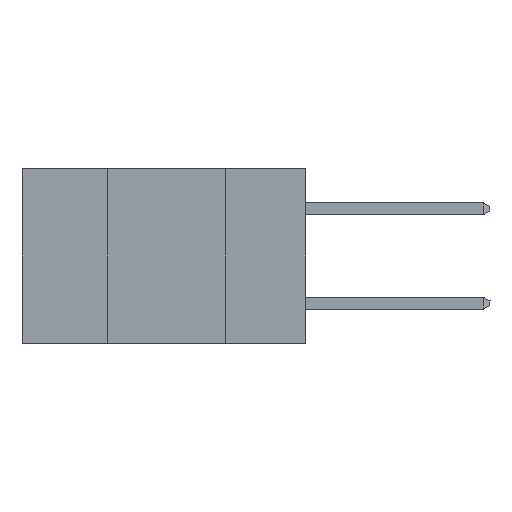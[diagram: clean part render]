
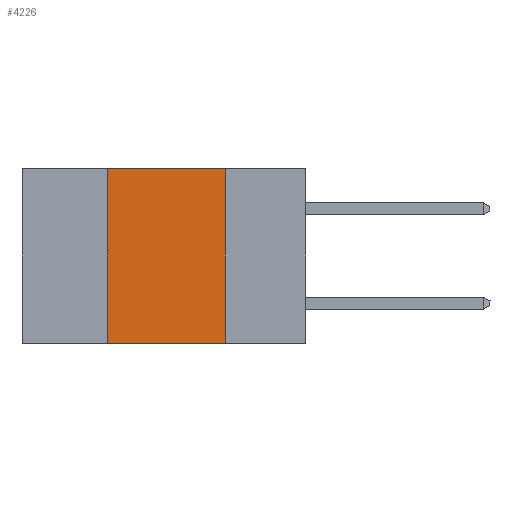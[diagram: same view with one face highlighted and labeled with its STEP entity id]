
A CAD part, left-side view. The second image highlights one B-rep face of the part: STEP entity #4226.
In plain terms, the highlighted planar face has unit normal (-1, 0, 0).
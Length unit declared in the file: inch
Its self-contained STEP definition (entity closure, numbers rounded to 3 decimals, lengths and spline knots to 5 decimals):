
#1037 = CARTESIAN_POINT ( 'NONE',  ( 0., 0.17, 0. ) ) ;
#1334 = ORIENTED_EDGE ( 'NONE', *, *, #5843, .T. ) ;
#3464 = LINE ( 'NONE', #20266, #15137 ) ;
#4077 = LINE ( 'NONE', #15122, #23071 ) ;
#4226 = ADVANCED_FACE ( 'NONE', ( #20405 ), #10790, .F. ) ;
#4358 = LINE ( 'NONE', #14824, #25282 ) ;
#4755 = VERTEX_POINT ( 'NONE', #24695 ) ;
#4991 = CARTESIAN_POINT ( 'NONE',  ( 0., 0.42, -0.37 ) ) ;
#5843 = EDGE_CURVE ( 'NONE', #17392, #4755, #12182, .T. ) ;
#6751 = VECTOR ( 'NONE', #26290, 39.37008 ) ;
#8142 = DIRECTION ( 'NONE',  ( 0., 0., 1. ) ) ;
#9183 = CARTESIAN_POINT ( 'NONE',  ( 0., 0.6, -0.37 ) ) ;
#10131 = EDGE_CURVE ( 'NONE', #29960, #4755, #4358, .T. ) ;
#10790 = PLANE ( 'NONE',  #16932 ) ;
#12182 = LINE ( 'NONE', #9183, #6751 ) ;
#12413 = DIRECTION ( 'NONE',  ( 0., 0., -1. ) ) ;
#12673 = EDGE_CURVE ( 'NONE', #17392, #29295, #3464, .T. ) ;
#14824 = CARTESIAN_POINT ( 'NONE',  ( 0., 0.17, 0. ) ) ;
#15122 = CARTESIAN_POINT ( 'NONE',  ( 0., 0.6, 0. ) ) ;
#15137 = VECTOR ( 'NONE', #8142, 39.37008 ) ;
#15389 = EDGE_CURVE ( 'NONE', #29295, #29960, #4077, .T. ) ;
#16932 = AXIS2_PLACEMENT_3D ( 'NONE', #29563, #25212, #27779 ) ;
#17300 = EDGE_LOOP ( 'NONE', ( #28672, #28970, #20698, #1334 ) ) ;
#17392 = VERTEX_POINT ( 'NONE', #4991 ) ;
#18484 = CARTESIAN_POINT ( 'NONE',  ( 0., 0.42, 0. ) ) ;
#20266 = CARTESIAN_POINT ( 'NONE',  ( 0., 0.42, 0. ) ) ;
#20405 = FACE_OUTER_BOUND ( 'NONE', #17300, .T. ) ;
#20698 = ORIENTED_EDGE ( 'NONE', *, *, #12673, .F. ) ;
#23071 = VECTOR ( 'NONE', #25623, 39.37008 ) ;
#24695 = CARTESIAN_POINT ( 'NONE',  ( 0., 0.17, -0.37 ) ) ;
#25212 = DIRECTION ( 'NONE',  ( 1., 0., 0. ) ) ;
#25282 = VECTOR ( 'NONE', #12413, 39.37008 ) ;
#25623 = DIRECTION ( 'NONE',  ( 0., -1., 0. ) ) ;
#26290 = DIRECTION ( 'NONE',  ( 0., -1., 0. ) ) ;
#27779 = DIRECTION ( 'NONE',  ( 0., 0., -1. ) ) ;
#28672 = ORIENTED_EDGE ( 'NONE', *, *, #10131, .F. ) ;
#28970 = ORIENTED_EDGE ( 'NONE', *, *, #15389, .F. ) ;
#29295 = VERTEX_POINT ( 'NONE', #18484 ) ;
#29563 = CARTESIAN_POINT ( 'NONE',  ( 0., 0.6, 0. ) ) ;
#29960 = VERTEX_POINT ( 'NONE', #1037 ) ;
